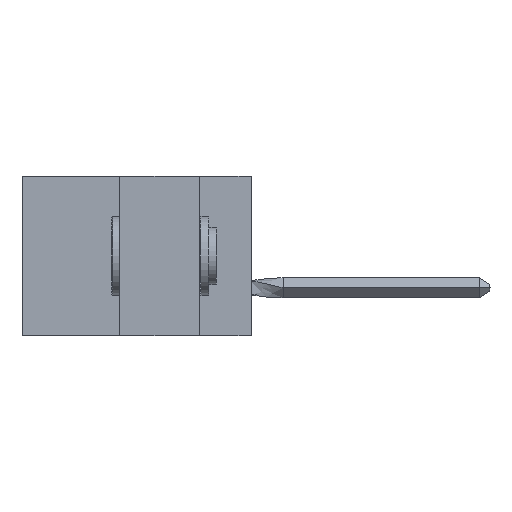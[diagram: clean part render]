
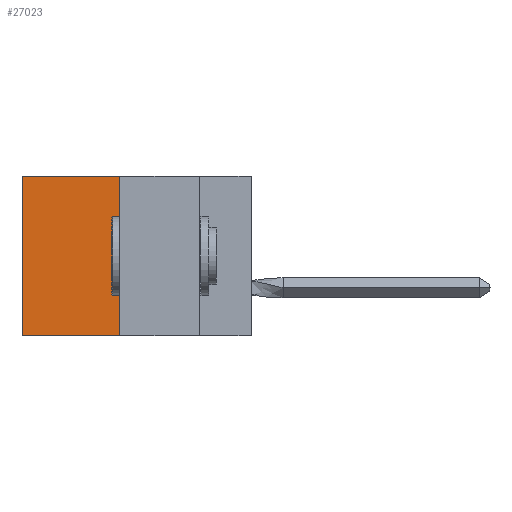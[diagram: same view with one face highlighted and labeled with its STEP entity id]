
A CAD part, left-side view. The second image highlights one B-rep face of the part: STEP entity #27023.
In plain terms, the highlighted planar face has unit normal (-1, 0, 0).
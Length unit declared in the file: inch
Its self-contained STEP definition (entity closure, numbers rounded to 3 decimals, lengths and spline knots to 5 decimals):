
#651 = CARTESIAN_POINT ( 'NONE',  ( 0.305, 0.413, -0.5 ) ) ;
#1369 = DIRECTION ( 'NONE',  ( 1., 0., 0. ) ) ;
#2195 = AXIS2_PLACEMENT_3D ( 'NONE', #8255, #1369, #3423 ) ;
#3423 = DIRECTION ( 'NONE',  ( 0., 0., -1. ) ) ;
#3988 = CARTESIAN_POINT ( 'NONE',  ( 0.305, 0.72, -0.5 ) ) ;
#5561 = DIRECTION ( 'NONE',  ( 0., 0., -1. ) ) ;
#6740 = DIRECTION ( 'NONE',  ( 0., 1., 0. ) ) ;
#7660 = DIRECTION ( 'NONE',  ( 0., 0., -1. ) ) ;
#8255 = CARTESIAN_POINT ( 'NONE',  ( 0.305, 0.413, -0.5 ) ) ;
#9009 = LINE ( 'NONE', #17572, #29974 ) ;
#9482 = LINE ( 'NONE', #22096, #26716 ) ;
#9561 = ORIENTED_EDGE ( 'NONE', *, *, #21493, .T. ) ;
#9640 = CARTESIAN_POINT ( 'NONE',  ( 0.305, 0.413, -0.5 ) ) ;
#10377 = DIRECTION ( 'NONE',  ( 0., 1., 0. ) ) ;
#11517 = VECTOR ( 'NONE', #6740, 39.37008 ) ;
#12988 = CARTESIAN_POINT ( 'NONE',  ( 0.305, 0.72, 0. ) ) ;
#13727 = VERTEX_POINT ( 'NONE', #28762 ) ;
#14406 = EDGE_CURVE ( 'NONE', #13727, #17003, #9009, .T. ) ;
#17003 = VERTEX_POINT ( 'NONE', #9640 ) ;
#17572 = CARTESIAN_POINT ( 'NONE',  ( 0.305, 0.413, -0.5 ) ) ;
#18133 = ORIENTED_EDGE ( 'NONE', *, *, #14406, .F. ) ;
#18425 = EDGE_LOOP ( 'NONE', ( #9561, #27471, #18133, #18992 ) ) ;
#18992 = ORIENTED_EDGE ( 'NONE', *, *, #25087, .T. ) ;
#19358 = LINE ( 'NONE', #27852, #11517 ) ;
#21493 = EDGE_CURVE ( 'NONE', #27046, #22199, #9482, .T. ) ;
#22096 = CARTESIAN_POINT ( 'NONE',  ( 0.305, 0.72, -0.5 ) ) ;
#22199 = VERTEX_POINT ( 'NONE', #3988 ) ;
#23363 = EDGE_CURVE ( 'NONE', #17003, #22199, #24507, .T. ) ;
#24507 = LINE ( 'NONE', #651, #25617 ) ;
#25087 = EDGE_CURVE ( 'NONE', #13727, #27046, #19358, .T. ) ;
#25617 = VECTOR ( 'NONE', #10377, 39.37008 ) ;
#26716 = VECTOR ( 'NONE', #7660, 39.37008 ) ;
#27023 = ADVANCED_FACE ( 'NONE', ( #28171 ), #27595, .F. ) ;
#27046 = VERTEX_POINT ( 'NONE', #12988 ) ;
#27471 = ORIENTED_EDGE ( 'NONE', *, *, #23363, .F. ) ;
#27595 = PLANE ( 'NONE',  #2195 ) ;
#27852 = CARTESIAN_POINT ( 'NONE',  ( 0.305, 0.413, 0. ) ) ;
#28171 = FACE_OUTER_BOUND ( 'NONE', #18425, .T. ) ;
#28762 = CARTESIAN_POINT ( 'NONE',  ( 0.305, 0.413, 0. ) ) ;
#29974 = VECTOR ( 'NONE', #5561, 39.37008 ) ;
